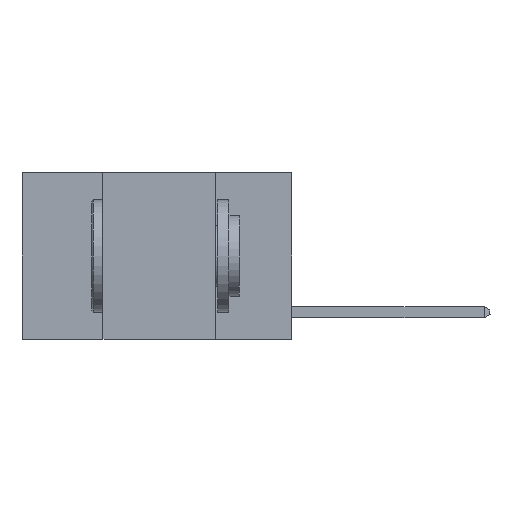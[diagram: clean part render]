
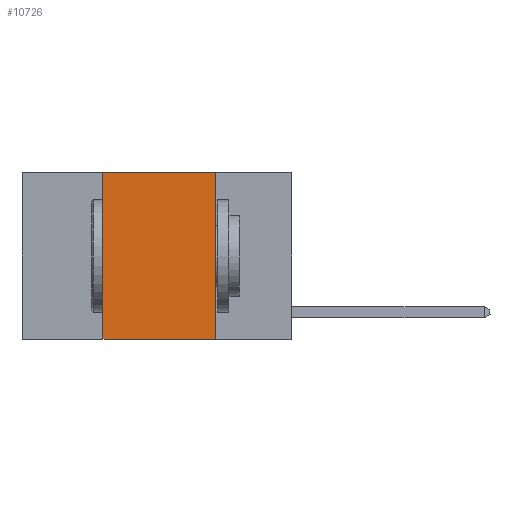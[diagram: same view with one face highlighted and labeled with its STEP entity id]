
A CAD part, left-side view. The second image highlights one B-rep face of the part: STEP entity #10726.
In plain terms, the highlighted planar face has unit normal (-1, 0, 0).
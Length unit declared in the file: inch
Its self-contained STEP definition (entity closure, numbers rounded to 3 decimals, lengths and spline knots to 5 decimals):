
#282 = CARTESIAN_POINT ( 'NONE',  ( 0., 0.17, -0.37 ) ) ;
#537 = ORIENTED_EDGE ( 'NONE', *, *, #15909, .F. ) ;
#759 = DIRECTION ( 'NONE',  ( 0., -1., 0. ) ) ;
#2258 = ORIENTED_EDGE ( 'NONE', *, *, #16228, .F. ) ;
#2724 = DIRECTION ( 'NONE',  ( 0., 0., -1. ) ) ;
#4424 = CARTESIAN_POINT ( 'NONE',  ( 0., 0.17, 0. ) ) ;
#5324 = AXIS2_PLACEMENT_3D ( 'NONE', #14783, #5897, #12079 ) ;
#5371 = VERTEX_POINT ( 'NONE', #282 ) ;
#5818 = PLANE ( 'NONE',  #5324 ) ;
#5897 = DIRECTION ( 'NONE',  ( 1., 0., 0. ) ) ;
#6017 = VERTEX_POINT ( 'NONE', #10494 ) ;
#6653 = EDGE_CURVE ( 'NONE', #6017, #15712, #15584, .T. ) ;
#7889 = CARTESIAN_POINT ( 'NONE',  ( 0., 0.42, 0. ) ) ;
#8714 = EDGE_CURVE ( 'NONE', #15173, #5371, #9391, .T. ) ;
#9235 = DIRECTION ( 'NONE',  ( 0., 0., 1. ) ) ;
#9391 = LINE ( 'NONE', #15776, #12220 ) ;
#9401 = VECTOR ( 'NONE', #9235, 39.37008 ) ;
#9409 = EDGE_LOOP ( 'NONE', ( #537, #10036, #2258, #15311 ) ) ;
#10036 = ORIENTED_EDGE ( 'NONE', *, *, #6653, .F. ) ;
#10360 = DIRECTION ( 'NONE',  ( 0., -1., 0. ) ) ;
#10494 = CARTESIAN_POINT ( 'NONE',  ( 0., 0.42, 0. ) ) ;
#10726 = ADVANCED_FACE ( 'NONE', ( #10908 ), #5818, .F. ) ;
#10766 = LINE ( 'NONE', #4424, #12615 ) ;
#10908 = FACE_OUTER_BOUND ( 'NONE', #9409, .T. ) ;
#12079 = DIRECTION ( 'NONE',  ( 0., 0., -1. ) ) ;
#12220 = VECTOR ( 'NONE', #759, 39.37008 ) ;
#12351 = VECTOR ( 'NONE', #10360, 39.37008 ) ;
#12615 = VECTOR ( 'NONE', #2724, 39.37008 ) ;
#12651 = CARTESIAN_POINT ( 'NONE',  ( 0., 0.42, -0.37 ) ) ;
#13019 = LINE ( 'NONE', #7889, #9401 ) ;
#14783 = CARTESIAN_POINT ( 'NONE',  ( 0., 0.6, 0. ) ) ;
#15173 = VERTEX_POINT ( 'NONE', #12651 ) ;
#15311 = ORIENTED_EDGE ( 'NONE', *, *, #8714, .T. ) ;
#15406 = CARTESIAN_POINT ( 'NONE',  ( 0., 0.17, 0. ) ) ;
#15422 = CARTESIAN_POINT ( 'NONE',  ( 0., 0.6, 0. ) ) ;
#15584 = LINE ( 'NONE', #15422, #12351 ) ;
#15712 = VERTEX_POINT ( 'NONE', #15406 ) ;
#15776 = CARTESIAN_POINT ( 'NONE',  ( 0., 0.6, -0.37 ) ) ;
#15909 = EDGE_CURVE ( 'NONE', #15712, #5371, #10766, .T. ) ;
#16228 = EDGE_CURVE ( 'NONE', #15173, #6017, #13019, .T. ) ;
